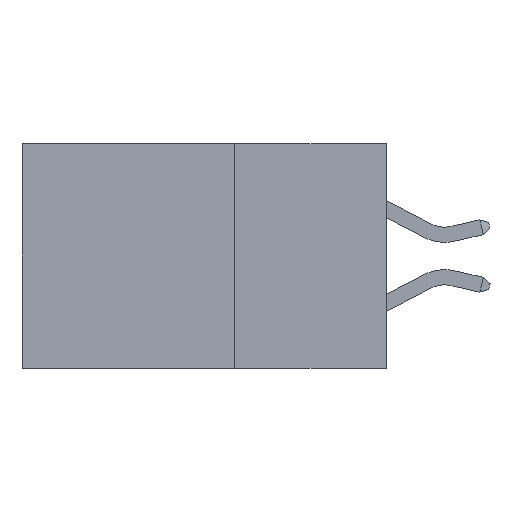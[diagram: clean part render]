
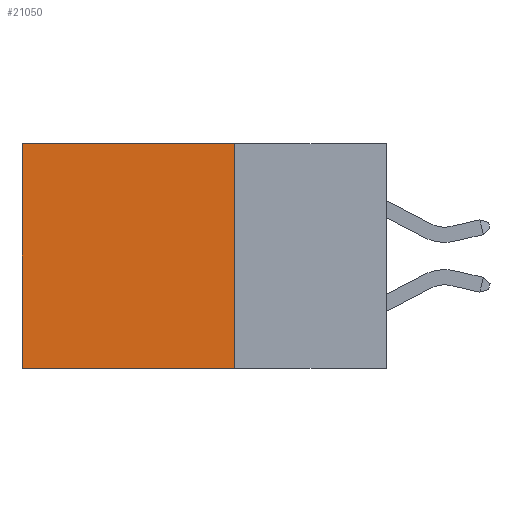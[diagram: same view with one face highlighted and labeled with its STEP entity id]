
A CAD part, left-side view. The second image highlights one B-rep face of the part: STEP entity #21050.
In plain terms, the highlighted planar face has unit normal (-1, 0, 0).
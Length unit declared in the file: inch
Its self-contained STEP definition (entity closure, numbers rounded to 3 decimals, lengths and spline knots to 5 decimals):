
#534 = VERTEX_POINT ( 'NONE', #7262 ) ;
#1151 = DIRECTION ( 'NONE',  ( 0., 0., -1. ) ) ;
#1263 = AXIS2_PLACEMENT_3D ( 'NONE', #18502, #16820, #1151 ) ;
#1450 = ORIENTED_EDGE ( 'NONE', *, *, #14021, .F. ) ;
#2199 = EDGE_CURVE ( 'NONE', #19412, #10003, #2474, .T. ) ;
#2474 = LINE ( 'NONE', #13868, #11127 ) ;
#3080 = FACE_OUTER_BOUND ( 'NONE', #10927, .T. ) ;
#3800 = EDGE_CURVE ( 'NONE', #19412, #534, #8895, .T. ) ;
#4710 = CARTESIAN_POINT ( 'NONE',  ( 0.298, 0.25, 0. ) ) ;
#5279 = CARTESIAN_POINT ( 'NONE',  ( 0.298, 0.25, -0.37 ) ) ;
#5466 = DIRECTION ( 'NONE',  ( 0., 1., 0. ) ) ;
#5739 = ORIENTED_EDGE ( 'NONE', *, *, #2199, .F. ) ;
#5791 = VECTOR ( 'NONE', #22168, 39.37008 ) ;
#6146 = ORIENTED_EDGE ( 'NONE', *, *, #8774, .T. ) ;
#7262 = CARTESIAN_POINT ( 'NONE',  ( 0.298, 0.6, 0. ) ) ;
#8774 = EDGE_CURVE ( 'NONE', #534, #10604, #16816, .T. ) ;
#8808 = ORIENTED_EDGE ( 'NONE', *, *, #3800, .T. ) ;
#8895 = LINE ( 'NONE', #13422, #17670 ) ;
#10003 = VERTEX_POINT ( 'NONE', #18565 ) ;
#10604 = VERTEX_POINT ( 'NONE', #17255 ) ;
#10927 = EDGE_LOOP ( 'NONE', ( #6146, #1450, #5739, #8808 ) ) ;
#11127 = VECTOR ( 'NONE', #20859, 39.37008 ) ;
#12052 = CARTESIAN_POINT ( 'NONE',  ( 0.298, 0.6, 0. ) ) ;
#13058 = PLANE ( 'NONE',  #1263 ) ;
#13422 = CARTESIAN_POINT ( 'NONE',  ( 0.298, 0.25, 0. ) ) ;
#13601 = DIRECTION ( 'NONE',  ( 0., 1., 0. ) ) ;
#13868 = CARTESIAN_POINT ( 'NONE',  ( 0.298, 0.25, 0. ) ) ;
#14021 = EDGE_CURVE ( 'NONE', #10003, #10604, #17899, .T. ) ;
#16816 = LINE ( 'NONE', #12052, #5791 ) ;
#16820 = DIRECTION ( 'NONE',  ( 1., 0., 0. ) ) ;
#17255 = CARTESIAN_POINT ( 'NONE',  ( 0.298, 0.6, -0.37 ) ) ;
#17670 = VECTOR ( 'NONE', #5466, 39.37008 ) ;
#17899 = LINE ( 'NONE', #5279, #21944 ) ;
#18502 = CARTESIAN_POINT ( 'NONE',  ( 0.298, 0.25, 0. ) ) ;
#18565 = CARTESIAN_POINT ( 'NONE',  ( 0.298, 0.25, -0.37 ) ) ;
#19412 = VERTEX_POINT ( 'NONE', #4710 ) ;
#20859 = DIRECTION ( 'NONE',  ( 0., 0., -1. ) ) ;
#21050 = ADVANCED_FACE ( 'NONE', ( #3080 ), #13058, .F. ) ;
#21944 = VECTOR ( 'NONE', #13601, 39.37008 ) ;
#22168 = DIRECTION ( 'NONE',  ( 0., 0., -1. ) ) ;
